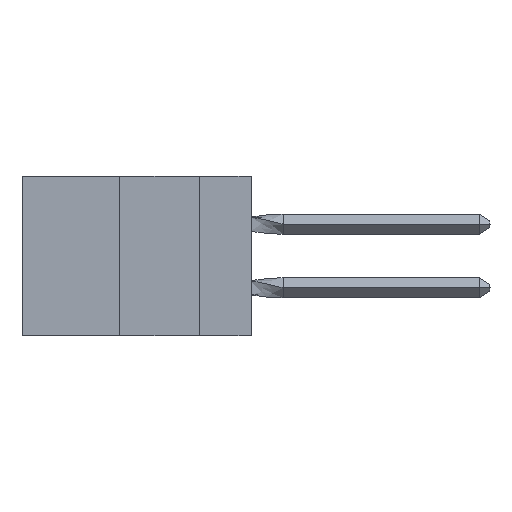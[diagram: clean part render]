
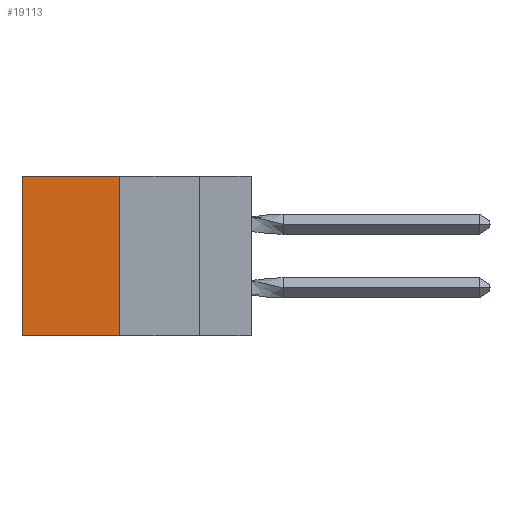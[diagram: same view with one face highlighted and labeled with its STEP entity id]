
A CAD part, left-side view. The second image highlights one B-rep face of the part: STEP entity #19113.
In plain terms, the highlighted planar face has unit normal (-1, 0, 0).
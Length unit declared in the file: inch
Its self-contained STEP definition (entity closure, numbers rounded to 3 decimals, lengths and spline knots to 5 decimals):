
#1223 = CARTESIAN_POINT ( 'NONE',  ( 0.305, 0.72, 0. ) ) ;
#3189 = CARTESIAN_POINT ( 'NONE',  ( 0.305, 0.72, -0.5 ) ) ;
#4140 = AXIS2_PLACEMENT_3D ( 'NONE', #34111, #16777, #36999 ) ;
#4554 = DIRECTION ( 'NONE',  ( 0., 0., -1. ) ) ;
#4965 = CARTESIAN_POINT ( 'NONE',  ( 0.305, 0.413, 0. ) ) ;
#5043 = VECTOR ( 'NONE', #4554, 39.37008 ) ;
#5770 = CARTESIAN_POINT ( 'NONE',  ( 0.305, 0.413, -0.5 ) ) ;
#5854 = FACE_OUTER_BOUND ( 'NONE', #21416, .T. ) ;
#6270 = ORIENTED_EDGE ( 'NONE', *, *, #9203, .T. ) ;
#6513 = CARTESIAN_POINT ( 'NONE',  ( 0.305, 0.413, 0. ) ) ;
#6798 = LINE ( 'NONE', #35949, #18121 ) ;
#7486 = EDGE_CURVE ( 'NONE', #29509, #27092, #9003, .T. ) ;
#9003 = LINE ( 'NONE', #11067, #25287 ) ;
#9203 = EDGE_CURVE ( 'NONE', #26826, #29509, #34234, .T. ) ;
#10266 = DIRECTION ( 'NONE',  ( 0., 1., 0. ) ) ;
#10696 = VECTOR ( 'NONE', #26481, 39.37008 ) ;
#11067 = CARTESIAN_POINT ( 'NONE',  ( 0.305, 0.72, -0.5 ) ) ;
#12005 = ORIENTED_EDGE ( 'NONE', *, *, #21720, .F. ) ;
#13264 = ORIENTED_EDGE ( 'NONE', *, *, #18306, .F. ) ;
#15458 = LINE ( 'NONE', #36267, #5043 ) ;
#16777 = DIRECTION ( 'NONE',  ( 1., 0., 0. ) ) ;
#18121 = VECTOR ( 'NONE', #10266, 39.37008 ) ;
#18306 = EDGE_CURVE ( 'NONE', #19201, #27092, #6798, .T. ) ;
#19113 = ADVANCED_FACE ( 'NONE', ( #5854 ), #36515, .F. ) ;
#19201 = VERTEX_POINT ( 'NONE', #5770 ) ;
#21416 = EDGE_LOOP ( 'NONE', ( #26181, #13264, #12005, #6270 ) ) ;
#21720 = EDGE_CURVE ( 'NONE', #26826, #19201, #15458, .T. ) ;
#25210 = DIRECTION ( 'NONE',  ( 0., 0., -1. ) ) ;
#25287 = VECTOR ( 'NONE', #25210, 39.37008 ) ;
#26181 = ORIENTED_EDGE ( 'NONE', *, *, #7486, .T. ) ;
#26481 = DIRECTION ( 'NONE',  ( 0., 1., 0. ) ) ;
#26826 = VERTEX_POINT ( 'NONE', #4965 ) ;
#27092 = VERTEX_POINT ( 'NONE', #3189 ) ;
#29509 = VERTEX_POINT ( 'NONE', #1223 ) ;
#34111 = CARTESIAN_POINT ( 'NONE',  ( 0.305, 0.413, -0.5 ) ) ;
#34234 = LINE ( 'NONE', #6513, #10696 ) ;
#35949 = CARTESIAN_POINT ( 'NONE',  ( 0.305, 0.413, -0.5 ) ) ;
#36267 = CARTESIAN_POINT ( 'NONE',  ( 0.305, 0.413, -0.5 ) ) ;
#36515 = PLANE ( 'NONE',  #4140 ) ;
#36999 = DIRECTION ( 'NONE',  ( 0., 0., -1. ) ) ;
